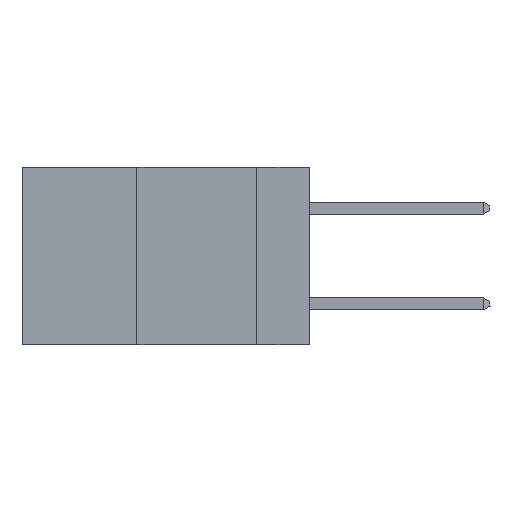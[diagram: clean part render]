
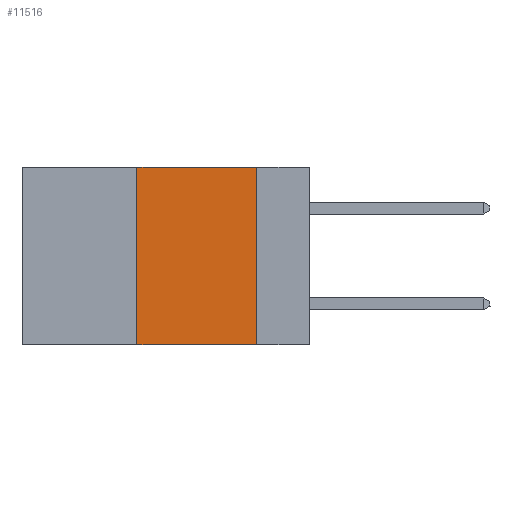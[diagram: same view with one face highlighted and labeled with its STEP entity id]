
A CAD part, left-side view. The second image highlights one B-rep face of the part: STEP entity #11516.
In plain terms, the highlighted planar face has unit normal (-1, 0, 0).
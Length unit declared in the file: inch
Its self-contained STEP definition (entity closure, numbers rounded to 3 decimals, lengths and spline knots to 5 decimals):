
#354 = DIRECTION ( 'NONE',  ( 0., 0., -1. ) ) ;
#741 = DIRECTION ( 'NONE',  ( 0., -1., 0. ) ) ;
#1301 = ORIENTED_EDGE ( 'NONE', *, *, #27287, .T. ) ;
#2599 = CARTESIAN_POINT ( 'NONE',  ( 0., 0.36, -0.37 ) ) ;
#2707 = DIRECTION ( 'NONE',  ( 1., 0., 0. ) ) ;
#2795 = VECTOR ( 'NONE', #741, 39.37008 ) ;
#3168 = FACE_OUTER_BOUND ( 'NONE', #26492, .T. ) ;
#4737 = LINE ( 'NONE', #14254, #19536 ) ;
#5478 = CARTESIAN_POINT ( 'NONE',  ( 0., 0.6, 0. ) ) ;
#6611 = VERTEX_POINT ( 'NONE', #20983 ) ;
#7520 = VECTOR ( 'NONE', #14523, 39.37008 ) ;
#7974 = LINE ( 'NONE', #5478, #20130 ) ;
#9163 = ORIENTED_EDGE ( 'NONE', *, *, #11012, .F. ) ;
#9640 = VERTEX_POINT ( 'NONE', #15244 ) ;
#10264 = EDGE_CURVE ( 'NONE', #12554, #9640, #4737, .T. ) ;
#11012 = EDGE_CURVE ( 'NONE', #20180, #6611, #19362, .T. ) ;
#11161 = ORIENTED_EDGE ( 'NONE', *, *, #22658, .F. ) ;
#11516 = ADVANCED_FACE ( 'NONE', ( #3168 ), #12704, .F. ) ;
#12554 = VERTEX_POINT ( 'NONE', #28288 ) ;
#12704 = PLANE ( 'NONE',  #15455 ) ;
#13257 = LINE ( 'NONE', #17941, #2795 ) ;
#14106 = DIRECTION ( 'NONE',  ( 0., 0., -1. ) ) ;
#14254 = CARTESIAN_POINT ( 'NONE',  ( 0., 0.11, 0. ) ) ;
#14523 = DIRECTION ( 'NONE',  ( 0., 0., 1. ) ) ;
#15244 = CARTESIAN_POINT ( 'NONE',  ( 0., 0.11, -0.37 ) ) ;
#15455 = AXIS2_PLACEMENT_3D ( 'NONE', #19446, #2707, #354 ) ;
#17505 = DIRECTION ( 'NONE',  ( 0., -1., 0. ) ) ;
#17723 = ORIENTED_EDGE ( 'NONE', *, *, #10264, .F. ) ;
#17941 = CARTESIAN_POINT ( 'NONE',  ( 0., 0.6, -0.37 ) ) ;
#19362 = LINE ( 'NONE', #28918, #7520 ) ;
#19446 = CARTESIAN_POINT ( 'NONE',  ( 0., 0.6, 0. ) ) ;
#19536 = VECTOR ( 'NONE', #14106, 39.37008 ) ;
#20130 = VECTOR ( 'NONE', #17505, 39.37008 ) ;
#20180 = VERTEX_POINT ( 'NONE', #2599 ) ;
#20983 = CARTESIAN_POINT ( 'NONE',  ( 0., 0.36, 0. ) ) ;
#22658 = EDGE_CURVE ( 'NONE', #6611, #12554, #7974, .T. ) ;
#26492 = EDGE_LOOP ( 'NONE', ( #17723, #11161, #9163, #1301 ) ) ;
#27287 = EDGE_CURVE ( 'NONE', #20180, #9640, #13257, .T. ) ;
#28288 = CARTESIAN_POINT ( 'NONE',  ( 0., 0.11, 0. ) ) ;
#28918 = CARTESIAN_POINT ( 'NONE',  ( 0., 0.36, 0. ) ) ;
